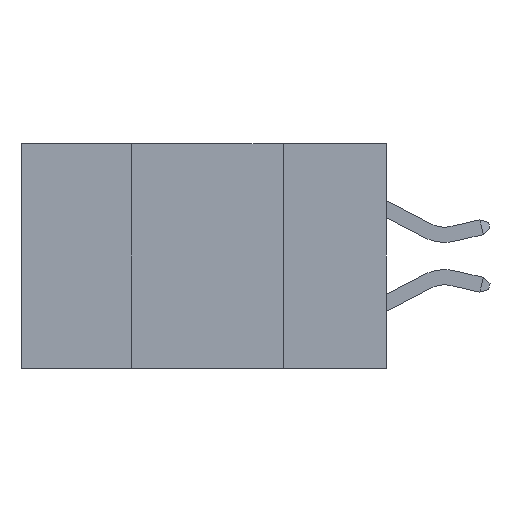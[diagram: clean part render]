
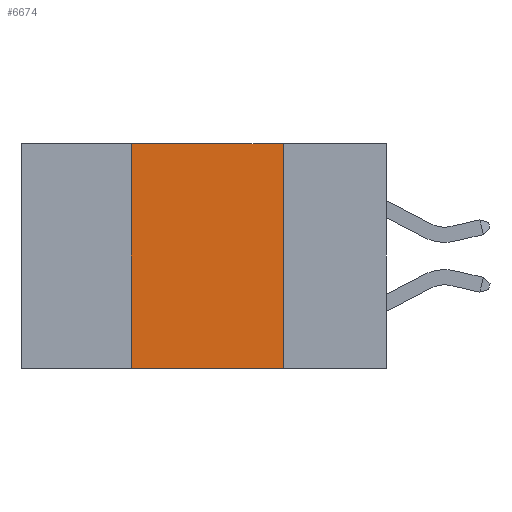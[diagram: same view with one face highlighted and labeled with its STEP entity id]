
A CAD part, left-side view. The second image highlights one B-rep face of the part: STEP entity #6674.
In plain terms, the highlighted planar face has unit normal (-1, 0, 0).
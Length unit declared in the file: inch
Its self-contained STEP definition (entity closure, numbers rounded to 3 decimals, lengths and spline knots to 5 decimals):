
#81 = VECTOR ( 'NONE', #2106, 39.37008 ) ;
#173 = PLANE ( 'NONE',  #8161 ) ;
#1079 = VECTOR ( 'NONE', #10048, 39.37008 ) ;
#1141 = DIRECTION ( 'NONE',  ( 0., 0., -1. ) ) ;
#1631 = EDGE_CURVE ( 'NONE', #8248, #5268, #2700, .T. ) ;
#1935 = ORIENTED_EDGE ( 'NONE', *, *, #4487, .F. ) ;
#2025 = CARTESIAN_POINT ( 'NONE',  ( 0., 0.17, 0. ) ) ;
#2075 = CARTESIAN_POINT ( 'NONE',  ( 0., 0.17, -0.37 ) ) ;
#2106 = DIRECTION ( 'NONE',  ( 0., -1., 0. ) ) ;
#2136 = LINE ( 'NONE', #2075, #7917 ) ;
#2166 = CARTESIAN_POINT ( 'NONE',  ( 0., 0.6, -0.37 ) ) ;
#2700 = LINE ( 'NONE', #9614, #4258 ) ;
#2952 = EDGE_CURVE ( 'NONE', #8502, #3238, #6475, .T. ) ;
#3238 = VERTEX_POINT ( 'NONE', #9871 ) ;
#3282 = ORIENTED_EDGE ( 'NONE', *, *, #2952, .T. ) ;
#3514 = ORIENTED_EDGE ( 'NONE', *, *, #5733, .F. ) ;
#4258 = VECTOR ( 'NONE', #9566, 39.37008 ) ;
#4487 = EDGE_CURVE ( 'NONE', #5268, #3238, #2136, .T. ) ;
#4580 = EDGE_LOOP ( 'NONE', ( #1935, #9555, #3514, #3282 ) ) ;
#5268 = VERTEX_POINT ( 'NONE', #2025 ) ;
#5733 = EDGE_CURVE ( 'NONE', #8502, #8248, #7233, .T. ) ;
#5814 = DIRECTION ( 'NONE',  ( 1., 0., 0. ) ) ;
#5910 = DIRECTION ( 'NONE',  ( 0., 0., -1. ) ) ;
#6475 = LINE ( 'NONE', #2166, #81 ) ;
#6674 = ADVANCED_FACE ( 'NONE', ( #8345 ), #173, .F. ) ;
#6912 = CARTESIAN_POINT ( 'NONE',  ( 0., 0.42, -0.37 ) ) ;
#7233 = LINE ( 'NONE', #7811, #1079 ) ;
#7811 = CARTESIAN_POINT ( 'NONE',  ( 0., 0.42, -0.37 ) ) ;
#7917 = VECTOR ( 'NONE', #5910, 39.37008 ) ;
#7985 = CARTESIAN_POINT ( 'NONE',  ( 0., 0.6, 0. ) ) ;
#8161 = AXIS2_PLACEMENT_3D ( 'NONE', #7985, #5814, #1141 ) ;
#8248 = VERTEX_POINT ( 'NONE', #8798 ) ;
#8345 = FACE_OUTER_BOUND ( 'NONE', #4580, .T. ) ;
#8502 = VERTEX_POINT ( 'NONE', #6912 ) ;
#8798 = CARTESIAN_POINT ( 'NONE',  ( 0., 0.42, 0. ) ) ;
#9555 = ORIENTED_EDGE ( 'NONE', *, *, #1631, .F. ) ;
#9566 = DIRECTION ( 'NONE',  ( 0., -1., 0. ) ) ;
#9614 = CARTESIAN_POINT ( 'NONE',  ( 0., 0.6, 0. ) ) ;
#9871 = CARTESIAN_POINT ( 'NONE',  ( 0., 0.17, -0.37 ) ) ;
#10048 = DIRECTION ( 'NONE',  ( 0., 0., 1. ) ) ;
